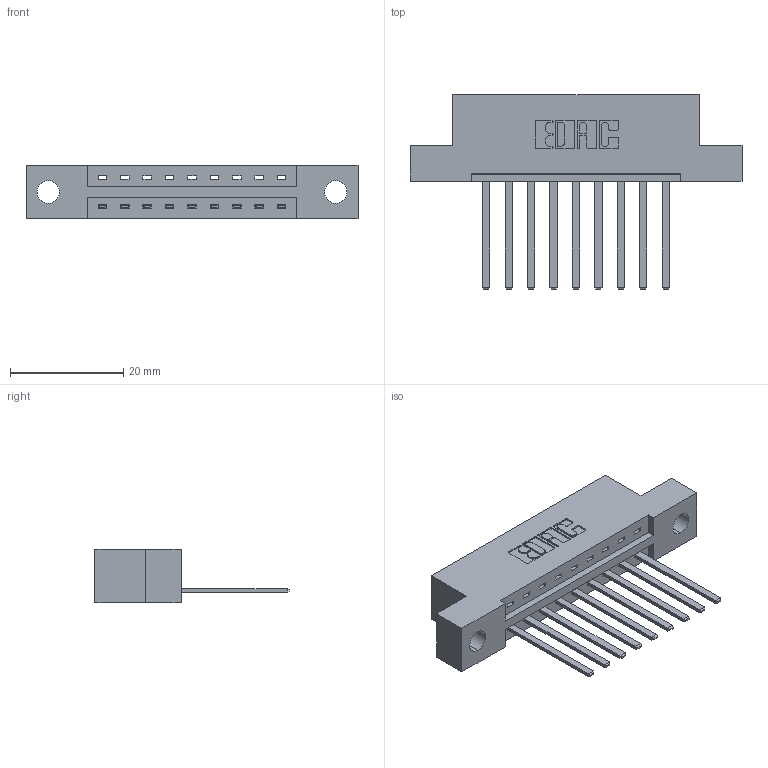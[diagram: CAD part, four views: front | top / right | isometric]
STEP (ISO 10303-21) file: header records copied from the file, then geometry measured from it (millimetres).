
FILE_DESCRIPTION (( 'STEP AP203' ), '1' );
FILE_NAME ('337-009-544-104.STEP', '2019-09-27T20:33:07', ( '' ), ( '' ), 'SwSTEP 2.0', 'SolidWorks 2016', '' );
FILE_SCHEMA (( 'CONFIG_CONTROL_DESIGN' ));
Length unit declared in the file: inch
Products named in the file (3): 345-292-001_345-293-144; 337-009-544-104; 337 Part_Flush Mounting Lugs - 0.156 Dia-TH
Assembly tree (10 placements, depth 2):
  337-009-544-104
    337 Part_Flush Mounting Lugs - 0.156 Dia-TH
    345-292-001_345-293-144  x9
Bounding box: 58.67 x 34.3 x 9.4 mm (x, y, z)
Volume: 5701.6 mm3; surface area: 5846.8 mm2
Topology: 10 solids, 10 shells, 618 faces, 1841 edges, 1214 vertices
Faces by surface type: plane 448, cylinder 170
Entity records: 10777 total; most frequent: CARTESIAN_POINT 1881, ORIENTED_EDGE 1826, DIRECTION 1647, EDGE_CURVE 913, LINE 789, VECTOR 789, VERTEX_POINT 606, AXIS2_PLACEMENT_3D 429
